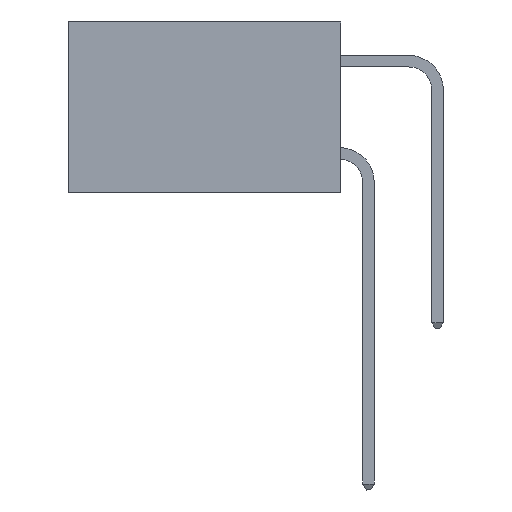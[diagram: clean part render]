
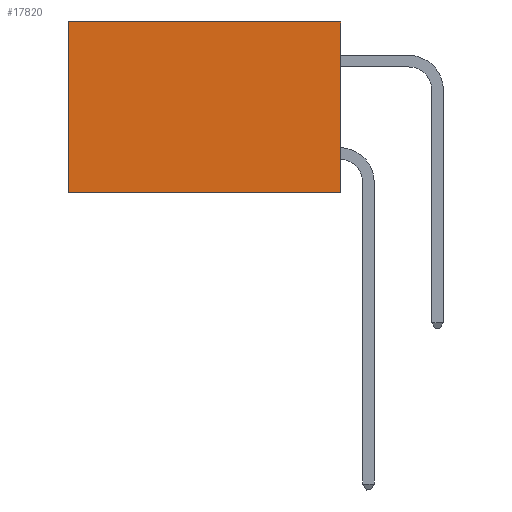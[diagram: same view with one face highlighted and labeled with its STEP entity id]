
A CAD part, left-side view. The second image highlights one B-rep face of the part: STEP entity #17820.
In plain terms, the highlighted planar face has unit normal (-1, 0, 0).
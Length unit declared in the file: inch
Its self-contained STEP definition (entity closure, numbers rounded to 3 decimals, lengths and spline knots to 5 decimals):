
#116 = ORIENTED_EDGE ( 'NONE', *, *, #2567, .F. ) ;
#285 = PLANE ( 'NONE',  #5583 ) ;
#566 = VERTEX_POINT ( 'NONE', #19645 ) ;
#2151 = DIRECTION ( 'NONE',  ( 0., 0., -1. ) ) ;
#2567 = EDGE_CURVE ( 'NONE', #16795, #14051, #8480, .T. ) ;
#2627 = CARTESIAN_POINT ( 'NONE',  ( 0.277, 0., 0. ) ) ;
#3152 = DIRECTION ( 'NONE',  ( 0., 0., -1. ) ) ;
#3190 = DIRECTION ( 'NONE',  ( 0., 0., -1. ) ) ;
#5583 = AXIS2_PLACEMENT_3D ( 'NONE', #13049, #13128, #2151 ) ;
#7610 = EDGE_LOOP ( 'NONE', ( #22401, #16501, #116, #15963 ) ) ;
#8323 = CARTESIAN_POINT ( 'NONE',  ( 0.277, 0., -0.37 ) ) ;
#8480 = LINE ( 'NONE', #8323, #13333 ) ;
#8721 = CARTESIAN_POINT ( 'NONE',  ( 0.277, 0., 0. ) ) ;
#8992 = LINE ( 'NONE', #19035, #12698 ) ;
#10002 = VERTEX_POINT ( 'NONE', #19901 ) ;
#11706 = DIRECTION ( 'NONE',  ( 0., 1., 0. ) ) ;
#12698 = VECTOR ( 'NONE', #11706, 39.37008 ) ;
#13049 = CARTESIAN_POINT ( 'NONE',  ( 0.277, 0., -0.37 ) ) ;
#13128 = DIRECTION ( 'NONE',  ( 1., 0., 0. ) ) ;
#13224 = EDGE_CURVE ( 'NONE', #566, #10002, #19502, .T. ) ;
#13333 = VECTOR ( 'NONE', #3152, 39.37008 ) ;
#14051 = VERTEX_POINT ( 'NONE', #23648 ) ;
#15462 = DIRECTION ( 'NONE',  ( 0., 1., 0. ) ) ;
#15963 = ORIENTED_EDGE ( 'NONE', *, *, #17994, .T. ) ;
#16039 = CARTESIAN_POINT ( 'NONE',  ( 0.277, 0.59, -0.37 ) ) ;
#16501 = ORIENTED_EDGE ( 'NONE', *, *, #17967, .F. ) ;
#16722 = FACE_OUTER_BOUND ( 'NONE', #7610, .T. ) ;
#16795 = VERTEX_POINT ( 'NONE', #8721 ) ;
#17599 = LINE ( 'NONE', #2627, #21961 ) ;
#17820 = ADVANCED_FACE ( 'NONE', ( #16722 ), #285, .F. ) ;
#17967 = EDGE_CURVE ( 'NONE', #14051, #10002, #8992, .T. ) ;
#17994 = EDGE_CURVE ( 'NONE', #16795, #566, #17599, .T. ) ;
#19035 = CARTESIAN_POINT ( 'NONE',  ( 0.277, 0., -0.37 ) ) ;
#19502 = LINE ( 'NONE', #16039, #23778 ) ;
#19645 = CARTESIAN_POINT ( 'NONE',  ( 0.277, 0.59, 0. ) ) ;
#19901 = CARTESIAN_POINT ( 'NONE',  ( 0.277, 0.59, -0.37 ) ) ;
#21961 = VECTOR ( 'NONE', #15462, 39.37008 ) ;
#22401 = ORIENTED_EDGE ( 'NONE', *, *, #13224, .T. ) ;
#23648 = CARTESIAN_POINT ( 'NONE',  ( 0.277, 0., -0.37 ) ) ;
#23778 = VECTOR ( 'NONE', #3190, 39.37008 ) ;
